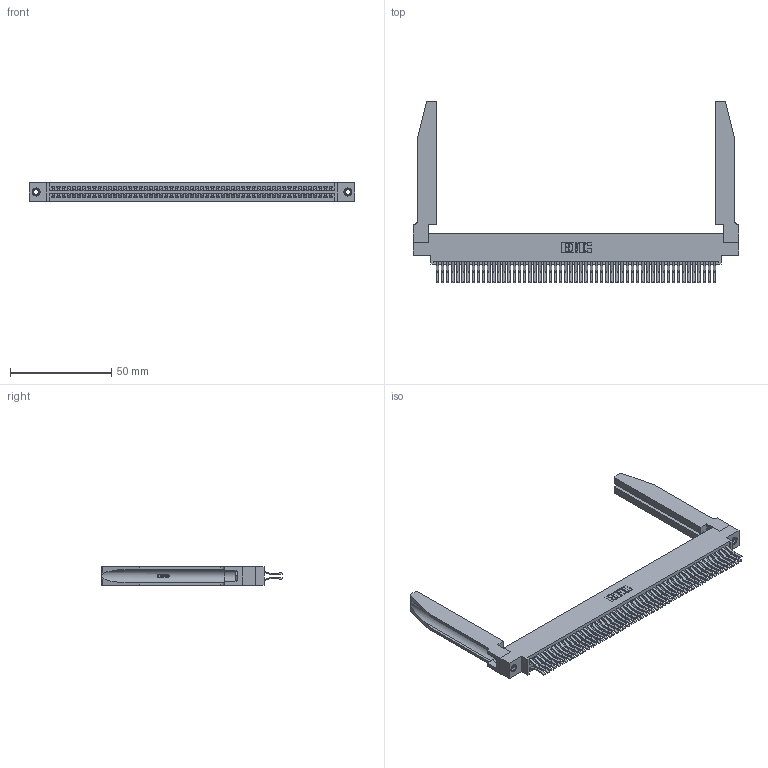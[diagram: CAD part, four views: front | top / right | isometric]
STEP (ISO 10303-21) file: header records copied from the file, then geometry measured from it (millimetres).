
FILE_DESCRIPTION (( 'STEP AP203' ), '1' );
FILE_NAME ('345-110-560-878.STEP', '2019-11-04T19:30:48', ( '' ), ( '' ), 'SwSTEP 2.0', 'SolidWorks 2016', '' );
FILE_SCHEMA (( 'CONFIG_CONTROL_DESIGN' ));
Length unit declared in the file: inch
Products named in the file (5): 345-110-560-878; 345-292-001_560 Tail; 345-220-078_345-220-078; 345 Part_0.170 Offset - 0.156 Dia-TH; 345-250-001_345-250-001-102
Assembly tree (115 placements, depth 2):
  345-110-560-878
    345 Part_0.170 Offset - 0.156 Dia-TH
    345-292-001_560 Tail  x110
    345-250-001_345-250-001-102  x2
    345-220-078_345-220-078  x2
Bounding box: 160.93 x 89.72 x 9.4 mm (x, y, z)
Volume: 24132.1 mm3; surface area: 33273.3 mm2
Topology: 115 solids, 115 shells, 6084 faces, 18011 edges, 11850 vertices
Faces by surface type: plane 3856, cylinder 2176, bspline 36, cone 12, torus 4
Entity records: 46364 total; most frequent: CARTESIAN_POINT 8679, ORIENTED_EDGE 7510, DIRECTION 6633, EDGE_CURVE 3755, LINE 3305, VECTOR 3305, VERTEX_POINT 2496, AXIS2_PLACEMENT_3D 1664
